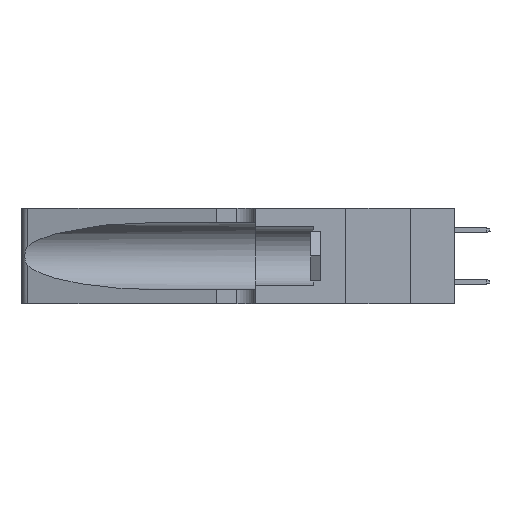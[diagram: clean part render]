
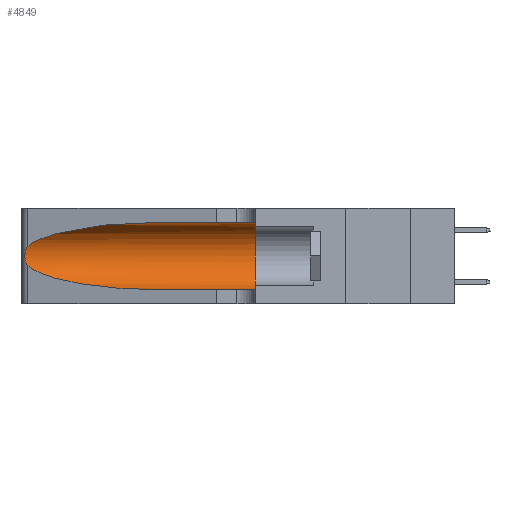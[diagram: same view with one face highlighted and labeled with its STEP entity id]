
A CAD part, left-side view. The second image highlights one B-rep face of the part: STEP entity #4849.
In plain terms, the highlighted cylindrical face has radius 3.308 mm (diameter 6.617 mm), a partial arc.
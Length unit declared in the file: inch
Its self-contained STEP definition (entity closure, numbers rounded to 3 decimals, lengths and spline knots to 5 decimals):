
#19 = EDGE_CURVE ( 'NONE', #33453, #25078, #20582, .T. ) ;
#590 = LINE ( 'NONE', #16472, #31083 ) ;
#2078 = CARTESIAN_POINT ( 'NONE',  ( 0.25854, 1.2359, 0.20912 ) ) ;
#2875 = CARTESIAN_POINT ( 'NONE',  ( 0.26017, 1.23833, 0.17102 ) ) ;
#4642 = DIRECTION ( 'NONE',  ( 0., 0., -1. ) ) ;
#4849 = ADVANCED_FACE ( 'NONE', ( #14289 ), #39491, .F. ) ;
#5005 = LINE ( 'NONE', #17154, #38166 ) ;
#5998 = EDGE_CURVE ( 'NONE', #29488, #33453, #18067, .T. ) ;
#6871 = ORIENTED_EDGE ( 'NONE', *, *, #36486, .T. ) ;
#7045 = CARTESIAN_POINT ( 'NONE',  ( 0.25487, 1.22718, 0.14631 ) ) ;
#7598 = CARTESIAN_POINT ( 'NONE',  ( 0.1305, 0.35, 0.05475 ) ) ;
#9174 = CARTESIAN_POINT ( 'NONE',  ( 0.26075, 1.23896, 0.178 ) ) ;
#9487 = DIRECTION ( 'NONE',  ( 0., 1., 0. ) ) ;
#10223 = DIRECTION ( 'NONE',  ( 0., -1., 0. ) ) ;
#10754 = VERTEX_POINT ( 'NONE', #7598 ) ;
#14289 = FACE_OUTER_BOUND ( 'NONE', #36998, .T. ) ;
#14685 = CARTESIAN_POINT ( 'NONE',  ( 0.1305, 1.61858, 0.185 ) ) ;
#14821 = CARTESIAN_POINT ( 'NONE',  ( 0.25789, 1.23486, 0.15765 ) ) ;
#15433 = CARTESIAN_POINT ( 'NONE',  ( 0.25487, 1.22718, 0.22369 ) ) ;
#16366 = CARTESIAN_POINT ( 'NONE',  ( 0.18966, 0.96281, 0.31525 ) ) ;
#16472 = CARTESIAN_POINT ( 'NONE',  ( 0.1305, 1.61858, 0.05475 ) ) ;
#16497 = VERTEX_POINT ( 'NONE', #27604 ) ;
#16857 = EDGE_CURVE ( 'NONE', #29488, #27926, #5005, .T. ) ;
#16955 = ORIENTED_EDGE ( 'NONE', *, *, #16857, .F. ) ;
#17154 = CARTESIAN_POINT ( 'NONE',  ( 0.1305, 1.61858, 0.31525 ) ) ;
#18067 =( BOUNDED_CURVE ( )  B_SPLINE_CURVE ( 3, ( #25967, #16366, #32023, #22634 ),
 .UNSPECIFIED., .F., .T. ) 
 B_SPLINE_CURVE_WITH_KNOTS ( ( 4, 4 ),
 ( 1.5708, 2.84003 ),
 .UNSPECIFIED. ) 
 CURVE ( )  GEOMETRIC_REPRESENTATION_ITEM ( )  RATIONAL_B_SPLINE_CURVE ( ( 1., 0.87, 0.87, 1. ) ) 
 REPRESENTATION_ITEM ( '' )  );
#18227 = AXIS2_PLACEMENT_3D ( 'NONE', #38852, #9487, #19080 ) ;
#18753 = CARTESIAN_POINT ( 'NONE',  ( 0.25856, 1.23593, 0.16098 ) ) ;
#18757 = DIRECTION ( 'NONE',  ( 0., -1., 0. ) ) ;
#19080 = DIRECTION ( 'NONE',  ( 0., 0., 1. ) ) ;
#19296 = ORIENTED_EDGE ( 'NONE', *, *, #27751, .T. ) ;
#19620 = CARTESIAN_POINT ( 'NONE',  ( 0.2373, 1.15595, 0.08982 ) ) ;
#20582 = B_SPLINE_CURVE_WITH_KNOTS ( 'NONE', 3,
 ( #15433, #25050, #40035, #27350, #2078, #40836, #37733, #9174, #2875, #18753, #14821, #27547, #40224, #37928 ),
 .UNSPECIFIED., .F., .F.,
 ( 4, 2, 2, 2, 2, 2, 4 ),
 ( 0., 0.00027, 0.00053, 0.00107, 0.0016, 0.00187, 0.00214 ),
 .UNSPECIFIED. ) ;
#20890 = CIRCLE ( 'NONE', #18227, 0.13025 ) ;
#21648 = CARTESIAN_POINT ( 'NONE',  ( 0.25487, 1.22718, 0.22369 ) ) ;
#21867 = ORIENTED_EDGE ( 'NONE', *, *, #29935, .F. ) ;
#22183 = AXIS2_PLACEMENT_3D ( 'NONE', #14685, #40095, #4642 ) ;
#22634 = CARTESIAN_POINT ( 'NONE',  ( 0.25487, 1.22718, 0.22369 ) ) ;
#22763 = CARTESIAN_POINT ( 'NONE',  ( 0.18966, 0.96281, 0.05475 ) ) ;
#23401 = CARTESIAN_POINT ( 'NONE',  ( 0.1305, 0.72297, 0.05475 ) ) ;
#25050 = CARTESIAN_POINT ( 'NONE',  ( 0.25555, 1.22994, 0.2215 ) ) ;
#25078 = VERTEX_POINT ( 'NONE', #7045 ) ;
#25967 = CARTESIAN_POINT ( 'NONE',  ( 0.1305, 0.72297, 0.31525 ) ) ;
#27350 = CARTESIAN_POINT ( 'NONE',  ( 0.25787, 1.23484, 0.2124 ) ) ;
#27547 = CARTESIAN_POINT ( 'NONE',  ( 0.25639, 1.23186, 0.15144 ) ) ;
#27604 = CARTESIAN_POINT ( 'NONE',  ( 0.1305, 0.72297, 0.05475 ) ) ;
#27751 = EDGE_CURVE ( 'NONE', #25078, #16497, #40194, .T. ) ;
#27926 = VERTEX_POINT ( 'NONE', #33998 ) ;
#28746 = CARTESIAN_POINT ( 'NONE',  ( 0.1305, 0.72297, 0.31525 ) ) ;
#29488 = VERTEX_POINT ( 'NONE', #28746 ) ;
#29935 = EDGE_CURVE ( 'NONE', #27926, #10754, #20890, .T. ) ;
#29982 = ORIENTED_EDGE ( 'NONE', *, *, #5998, .T. ) ;
#30664 = ORIENTED_EDGE ( 'NONE', *, *, #19, .T. ) ;
#31083 = VECTOR ( 'NONE', #10223, 39.37008 ) ;
#31323 = CARTESIAN_POINT ( 'NONE',  ( 0.25487, 1.22718, 0.14631 ) ) ;
#32023 = CARTESIAN_POINT ( 'NONE',  ( 0.2373, 1.15595, 0.28018 ) ) ;
#33453 = VERTEX_POINT ( 'NONE', #21648 ) ;
#33998 = CARTESIAN_POINT ( 'NONE',  ( 0.1305, 0.35, 0.31525 ) ) ;
#36486 = EDGE_CURVE ( 'NONE', #16497, #10754, #590, .T. ) ;
#36998 = EDGE_LOOP ( 'NONE', ( #29982, #30664, #19296, #6871, #21867, #16955 ) ) ;
#37733 = CARTESIAN_POINT ( 'NONE',  ( 0.26075, 1.23896, 0.19203 ) ) ;
#37928 = CARTESIAN_POINT ( 'NONE',  ( 0.25487, 1.22718, 0.14631 ) ) ;
#38166 = VECTOR ( 'NONE', #18757, 39.37008 ) ;
#38852 = CARTESIAN_POINT ( 'NONE',  ( 0.1305, 0.35, 0.185 ) ) ;
#39491 = CYLINDRICAL_SURFACE ( 'NONE', #22183, 0.13025 ) ;
#40035 = CARTESIAN_POINT ( 'NONE',  ( 0.25639, 1.23184, 0.21858 ) ) ;
#40095 = DIRECTION ( 'NONE',  ( 0., -1., 0. ) ) ;
#40194 =( BOUNDED_CURVE ( )  B_SPLINE_CURVE ( 3, ( #31323, #19620, #22763, #23401 ),
 .UNSPECIFIED., .F., .T. ) 
 B_SPLINE_CURVE_WITH_KNOTS ( ( 4, 4 ),
 ( 3.44316, 4.71239 ),
 .UNSPECIFIED. ) 
 CURVE ( )  GEOMETRIC_REPRESENTATION_ITEM ( )  RATIONAL_B_SPLINE_CURVE ( ( 1., 0.87, 0.87, 1. ) ) 
 REPRESENTATION_ITEM ( '' )  );
#40224 = CARTESIAN_POINT ( 'NONE',  ( 0.25555, 1.22993, 0.14849 ) ) ;
#40836 = CARTESIAN_POINT ( 'NONE',  ( 0.26018, 1.23835, 0.19895 ) ) ;
